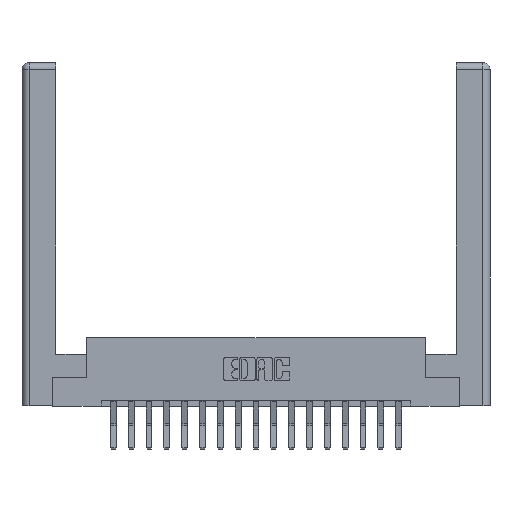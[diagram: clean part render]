
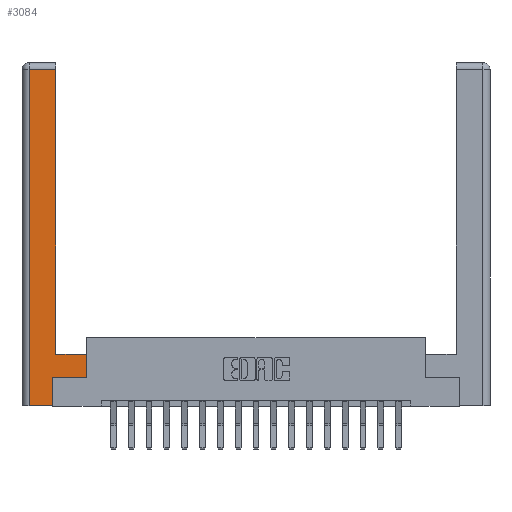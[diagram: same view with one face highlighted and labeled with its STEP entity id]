
A CAD part, top view. The second image highlights one B-rep face of the part: STEP entity #3084.
In plain terms, the highlighted planar face has unit normal (0, 0, 1).
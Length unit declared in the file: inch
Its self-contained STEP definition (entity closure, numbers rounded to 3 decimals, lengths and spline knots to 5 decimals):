
#127 = LINE ( 'NONE', #18621, #14902 ) ;
#560 = CARTESIAN_POINT ( 'NONE',  ( 0., 0., 0. ) ) ;
#727 = DIRECTION ( 'NONE',  ( 0., 1., 0. ) ) ;
#2129 = DIRECTION ( 'NONE',  ( 0., 1., 0. ) ) ;
#2203 = CARTESIAN_POINT ( 'NONE',  ( 0.565, 0.45, 0. ) ) ;
#2507 = CARTESIAN_POINT ( 'NONE',  ( 0.565, 0.245, 0. ) ) ;
#2568 = VECTOR ( 'NONE', #727, 39.37008 ) ;
#2858 = VERTEX_POINT ( 'NONE', #13652 ) ;
#3084 = ADVANCED_FACE ( 'NONE', ( #14480 ), #6593, .F. ) ;
#3114 = EDGE_CURVE ( 'NONE', #4475, #11741, #13560, .T. ) ;
#3232 = CARTESIAN_POINT ( 'NONE',  ( 0.0615, 2.94, 0. ) ) ;
#4038 = EDGE_CURVE ( 'NONE', #14212, #8382, #17178, .T. ) ;
#4437 = AXIS2_PLACEMENT_3D ( 'NONE', #560, #16979, #13724 ) ;
#4475 = VERTEX_POINT ( 'NONE', #3232 ) ;
#4924 = ORIENTED_EDGE ( 'NONE', *, *, #7451, .T. ) ;
#4935 = VERTEX_POINT ( 'NONE', #16633 ) ;
#5230 = VECTOR ( 'NONE', #14416, 39.37008 ) ;
#5397 = EDGE_CURVE ( 'NONE', #4935, #18970, #6665, .T. ) ;
#5689 = CARTESIAN_POINT ( 'NONE',  ( 0.295, 0.45, 0. ) ) ;
#5927 = LINE ( 'NONE', #8897, #11462 ) ;
#5942 = ORIENTED_EDGE ( 'NONE', *, *, #11758, .T. ) ;
#6147 = VECTOR ( 'NONE', #10272, 39.37008 ) ;
#6593 = PLANE ( 'NONE',  #4437 ) ;
#6665 = LINE ( 'NONE', #10930, #15930 ) ;
#6995 = VECTOR ( 'NONE', #18314, 39.37008 ) ;
#7341 = CARTESIAN_POINT ( 'NONE',  ( 0.295, 2.94, 0. ) ) ;
#7445 = LINE ( 'NONE', #16860, #6995 ) ;
#7451 = EDGE_CURVE ( 'NONE', #18970, #4475, #5927, .T. ) ;
#8367 = CARTESIAN_POINT ( 'NONE',  ( 0.565, 0.245, 0. ) ) ;
#8382 = VERTEX_POINT ( 'NONE', #15505 ) ;
#8897 = CARTESIAN_POINT ( 'NONE',  ( 0.0615, 2.94, 0. ) ) ;
#9177 = LINE ( 'NONE', #8367, #5230 ) ;
#9487 = EDGE_CURVE ( 'NONE', #11741, #18106, #7445, .T. ) ;
#9601 = CARTESIAN_POINT ( 'NONE',  ( 0.0615, 0., 0. ) ) ;
#9847 = CARTESIAN_POINT ( 'NONE',  ( 0.0615, 0., 0. ) ) ;
#10272 = DIRECTION ( 'NONE',  ( -1., 0., 0. ) ) ;
#10930 = CARTESIAN_POINT ( 'NONE',  ( 0.295, 3., 0. ) ) ;
#11462 = VECTOR ( 'NONE', #13743, 39.37008 ) ;
#11741 = VERTEX_POINT ( 'NONE', #9847 ) ;
#11758 = EDGE_CURVE ( 'NONE', #2858, #14212, #9177, .T. ) ;
#11804 = ORIENTED_EDGE ( 'NONE', *, *, #3114, .T. ) ;
#12459 = EDGE_CURVE ( 'NONE', #18106, #2858, #127, .T. ) ;
#12602 = EDGE_LOOP ( 'NONE', ( #13835, #4924, #11804, #12708, #16450, #5942, #15073, #13337 ) ) ;
#12708 = ORIENTED_EDGE ( 'NONE', *, *, #9487, .T. ) ;
#13337 = ORIENTED_EDGE ( 'NONE', *, *, #18894, .T. ) ;
#13560 = LINE ( 'NONE', #9601, #14945 ) ;
#13652 = CARTESIAN_POINT ( 'NONE',  ( 0.265, 0.245, 0. ) ) ;
#13724 = DIRECTION ( 'NONE',  ( -1., 0., 0. ) ) ;
#13743 = DIRECTION ( 'NONE',  ( -1., 0., 0. ) ) ;
#13835 = ORIENTED_EDGE ( 'NONE', *, *, #5397, .T. ) ;
#14109 = DIRECTION ( 'NONE',  ( 0., -1., 0. ) ) ;
#14212 = VERTEX_POINT ( 'NONE', #2507 ) ;
#14416 = DIRECTION ( 'NONE',  ( 1., 0., 0. ) ) ;
#14480 = FACE_OUTER_BOUND ( 'NONE', #12602, .T. ) ;
#14902 = VECTOR ( 'NONE', #2129, 39.37008 ) ;
#14945 = VECTOR ( 'NONE', #14109, 39.37008 ) ;
#14948 = LINE ( 'NONE', #5689, #6147 ) ;
#15019 = CARTESIAN_POINT ( 'NONE',  ( 0.265, 0., 0. ) ) ;
#15073 = ORIENTED_EDGE ( 'NONE', *, *, #4038, .T. ) ;
#15505 = CARTESIAN_POINT ( 'NONE',  ( 0.565, 0.45, 0. ) ) ;
#15930 = VECTOR ( 'NONE', #18307, 39.37008 ) ;
#16450 = ORIENTED_EDGE ( 'NONE', *, *, #12459, .T. ) ;
#16633 = CARTESIAN_POINT ( 'NONE',  ( 0.295, 0.45, 0. ) ) ;
#16860 = CARTESIAN_POINT ( 'NONE',  ( 0.265, 0., 0. ) ) ;
#16979 = DIRECTION ( 'NONE',  ( 0., 0., -1. ) ) ;
#17178 = LINE ( 'NONE', #2203, #2568 ) ;
#18106 = VERTEX_POINT ( 'NONE', #15019 ) ;
#18307 = DIRECTION ( 'NONE',  ( 0., 1., 0. ) ) ;
#18314 = DIRECTION ( 'NONE',  ( 1., 0., 0. ) ) ;
#18621 = CARTESIAN_POINT ( 'NONE',  ( 0.265, 0.245, 0. ) ) ;
#18894 = EDGE_CURVE ( 'NONE', #8382, #4935, #14948, .T. ) ;
#18970 = VERTEX_POINT ( 'NONE', #7341 ) ;
